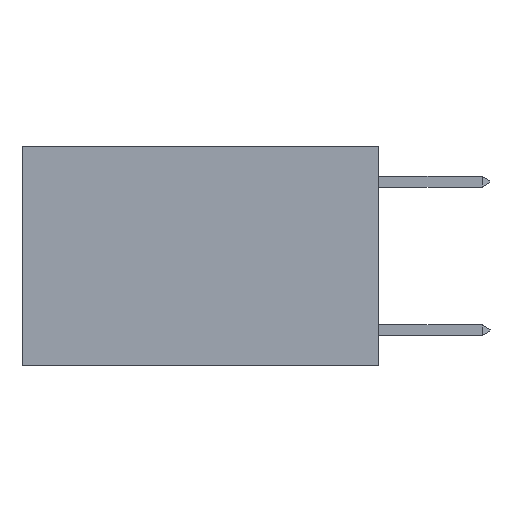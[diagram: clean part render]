
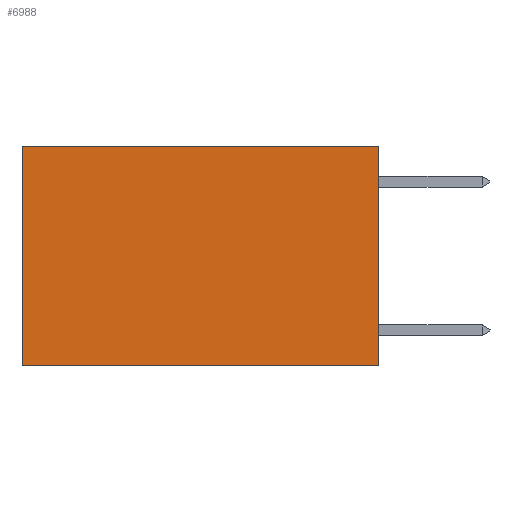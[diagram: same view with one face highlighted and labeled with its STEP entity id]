
A CAD part, left-side view. The second image highlights one B-rep face of the part: STEP entity #6988.
In plain terms, the highlighted planar face has unit normal (-1, 0, 0).
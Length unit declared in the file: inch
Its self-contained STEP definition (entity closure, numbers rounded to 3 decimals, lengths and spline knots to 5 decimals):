
#1513 = ORIENTED_EDGE ( 'NONE', *, *, #26040, .F. ) ;
#1773 = DIRECTION ( 'NONE',  ( 0., 0., -1. ) ) ;
#2030 = CARTESIAN_POINT ( 'NONE',  ( 0.2625, 0.6, -0.37 ) ) ;
#2350 = EDGE_CURVE ( 'NONE', #15814, #11218, #21444, .T. ) ;
#4294 = VECTOR ( 'NONE', #1773, 39.37008 ) ;
#5213 = CARTESIAN_POINT ( 'NONE',  ( 0.2625, 0., -0.37 ) ) ;
#5987 = FACE_OUTER_BOUND ( 'NONE', #12825, .T. ) ;
#5999 = ORIENTED_EDGE ( 'NONE', *, *, #7068, .T. ) ;
#6882 = VECTOR ( 'NONE', #8687, 39.37008 ) ;
#6988 = ADVANCED_FACE ( 'NONE', ( #5987 ), #12512, .F. ) ;
#7068 = EDGE_CURVE ( 'NONE', #11218, #16561, #23187, .T. ) ;
#8687 = DIRECTION ( 'NONE',  ( 0., 1., 0. ) ) ;
#9870 = VECTOR ( 'NONE', #23404, 39.37008 ) ;
#10263 = VECTOR ( 'NONE', #11109, 39.37008 ) ;
#11109 = DIRECTION ( 'NONE',  ( 0., 0., -1. ) ) ;
#11218 = VERTEX_POINT ( 'NONE', #13629 ) ;
#12512 = PLANE ( 'NONE',  #23400 ) ;
#12681 = CARTESIAN_POINT ( 'NONE',  ( 0.2625, 0., 0. ) ) ;
#12825 = EDGE_LOOP ( 'NONE', ( #5999, #1513, #18382, #23699 ) ) ;
#13629 = CARTESIAN_POINT ( 'NONE',  ( 0.2625, 0.6, 0. ) ) ;
#15250 = CARTESIAN_POINT ( 'NONE',  ( 0.2625, 0., 0. ) ) ;
#15814 = VERTEX_POINT ( 'NONE', #15250 ) ;
#16561 = VERTEX_POINT ( 'NONE', #2030 ) ;
#18382 = ORIENTED_EDGE ( 'NONE', *, *, #21223, .F. ) ;
#19371 = CARTESIAN_POINT ( 'NONE',  ( 0.2625, 0.6, 0. ) ) ;
#20545 = LINE ( 'NONE', #26237, #6882 ) ;
#21178 = CARTESIAN_POINT ( 'NONE',  ( 0.2625, 0., 0. ) ) ;
#21223 = EDGE_CURVE ( 'NONE', #15814, #24929, #27284, .T. ) ;
#21444 = LINE ( 'NONE', #21178, #9870 ) ;
#23187 = LINE ( 'NONE', #19371, #4294 ) ;
#23400 = AXIS2_PLACEMENT_3D ( 'NONE', #12681, #25996, #24186 ) ;
#23404 = DIRECTION ( 'NONE',  ( 0., 1., 0. ) ) ;
#23699 = ORIENTED_EDGE ( 'NONE', *, *, #2350, .T. ) ;
#24186 = DIRECTION ( 'NONE',  ( 0., 0., -1. ) ) ;
#24929 = VERTEX_POINT ( 'NONE', #5213 ) ;
#25996 = DIRECTION ( 'NONE',  ( 1., 0., 0. ) ) ;
#26040 = EDGE_CURVE ( 'NONE', #24929, #16561, #20545, .T. ) ;
#26237 = CARTESIAN_POINT ( 'NONE',  ( 0.2625, 0., -0.37 ) ) ;
#26241 = CARTESIAN_POINT ( 'NONE',  ( 0.2625, 0., 0. ) ) ;
#27284 = LINE ( 'NONE', #26241, #10263 ) ;
